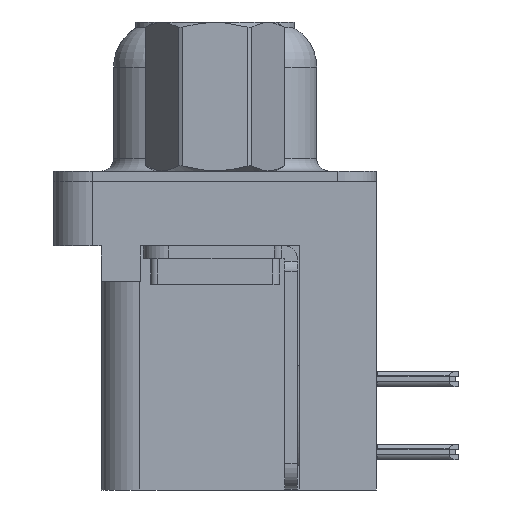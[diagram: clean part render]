
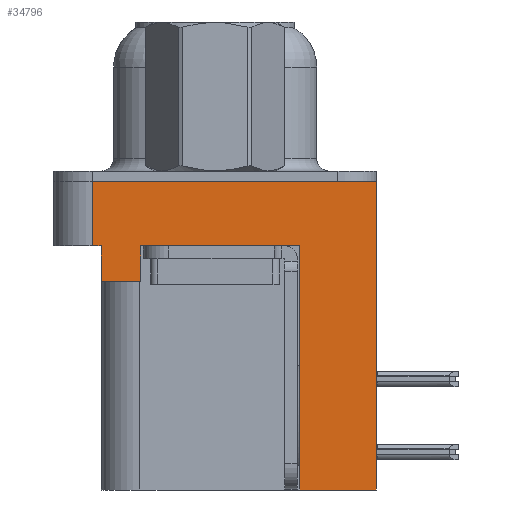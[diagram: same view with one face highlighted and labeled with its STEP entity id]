
A CAD part, left-side view. The second image highlights one B-rep face of the part: STEP entity #34796.
In plain terms, the highlighted planar face has unit normal (-1, 0, 0).
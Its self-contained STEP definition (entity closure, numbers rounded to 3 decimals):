
#203 = VECTOR ( 'NONE', #33293, 1000. ) ;
#661 = VERTEX_POINT ( 'NONE', #14032 ) ;
#701 = LINE ( 'NONE', #36045, #203 ) ;
#833 = LINE ( 'NONE', #17079, #24653 ) ;
#1160 = VERTEX_POINT ( 'NONE', #25653 ) ;
#1817 = VERTEX_POINT ( 'NONE', #3060 ) ;
#1868 = VECTOR ( 'NONE', #26045, 1000. ) ;
#1996 = VECTOR ( 'NONE', #5836, 1000. ) ;
#2116 = ORIENTED_EDGE ( 'NONE', *, *, #36443, .F. ) ;
#2632 = CARTESIAN_POINT ( 'NONE',  ( -3., 4.775, -2.5 ) ) ;
#3060 = CARTESIAN_POINT ( 'NONE',  ( -3., -3.295, -12. ) ) ;
#4125 = DIRECTION ( 'NONE',  ( 0., -1., 0. ) ) ;
#5106 = LINE ( 'NONE', #2632, #1996 ) ;
#5511 = DIRECTION ( 'NONE',  ( 0., 0., 1. ) ) ;
#5622 = ORIENTED_EDGE ( 'NONE', *, *, #32778, .F. ) ;
#5836 = DIRECTION ( 'NONE',  ( 0., 0., 1. ) ) ;
#6064 = FACE_OUTER_BOUND ( 'NONE', #20795, .T. ) ;
#6183 = DIRECTION ( 'NONE',  ( 0., 1., 0. ) ) ;
#6506 = VECTOR ( 'NONE', #8649, 1000. ) ;
#7012 = ORIENTED_EDGE ( 'NONE', *, *, #32223, .T. ) ;
#7039 = VERTEX_POINT ( 'NONE', #19351 ) ;
#7187 = VECTOR ( 'NONE', #5511, 1000. ) ;
#7406 = CARTESIAN_POINT ( 'NONE',  ( -3., -6.275, -2.5 ) ) ;
#8396 = LINE ( 'NONE', #28983, #18297 ) ;
#8625 = VERTEX_POINT ( 'NONE', #19706 ) ;
#8649 = DIRECTION ( 'NONE',  ( 0., 0., 1. ) ) ;
#9551 = VECTOR ( 'NONE', #12035, 1000. ) ;
#9947 = LINE ( 'NONE', #23900, #34202 ) ;
#11908 = CARTESIAN_POINT ( 'NONE',  ( -3., 2.895, -3.9 ) ) ;
#12035 = DIRECTION ( 'NONE',  ( 0., 1., 0. ) ) ;
#12467 = ORIENTED_EDGE ( 'NONE', *, *, #16066, .F. ) ;
#13062 = ORIENTED_EDGE ( 'NONE', *, *, #21105, .F. ) ;
#13386 = CARTESIAN_POINT ( 'NONE',  ( -3., -6.275, -12. ) ) ;
#14032 = CARTESIAN_POINT ( 'NONE',  ( -3., 4.425, -3.9 ) ) ;
#14175 = VECTOR ( 'NONE', #4125, 1000. ) ;
#14277 = ORIENTED_EDGE ( 'NONE', *, *, #25251, .F. ) ;
#14768 = CARTESIAN_POINT ( 'NONE',  ( -3., 4.425, -3.9 ) ) ;
#15149 = CARTESIAN_POINT ( 'NONE',  ( -3., -6.275, 0. ) ) ;
#15582 = ORIENTED_EDGE ( 'NONE', *, *, #23860, .T. ) ;
#16066 = EDGE_CURVE ( 'NONE', #28589, #8625, #5106, .T. ) ;
#16696 = ORIENTED_EDGE ( 'NONE', *, *, #24998, .T. ) ;
#17079 = CARTESIAN_POINT ( 'NONE',  ( -3., -3.295, -12. ) ) ;
#18297 = VECTOR ( 'NONE', #6183, 1000. ) ;
#19138 = LINE ( 'NONE', #15149, #14175 ) ;
#19351 = CARTESIAN_POINT ( 'NONE',  ( -3., 2.895, -3.9 ) ) ;
#19706 = CARTESIAN_POINT ( 'NONE',  ( -3., 4.775, 0. ) ) ;
#19817 = CARTESIAN_POINT ( 'NONE',  ( -3., -6.275, -2.5 ) ) ;
#20795 = EDGE_LOOP ( 'NONE', ( #13062, #12467, #32014, #25478, #14277, #16696, #15582, #5622, #2116, #7012 ) ) ;
#21105 = EDGE_CURVE ( 'NONE', #8625, #31920, #19138, .T. ) ;
#21643 = AXIS2_PLACEMENT_3D ( 'NONE', #7406, #30095, #27323 ) ;
#22109 = VERTEX_POINT ( 'NONE', #13386 ) ;
#22446 = LINE ( 'NONE', #19817, #7187 ) ;
#23860 = EDGE_CURVE ( 'NONE', #30116, #1160, #9947, .T. ) ;
#23900 = CARTESIAN_POINT ( 'NONE',  ( -3., -6.275, -2.5 ) ) ;
#24653 = VECTOR ( 'NONE', #28557, 1000. ) ;
#24717 = PLANE ( 'NONE',  #21643 ) ;
#24763 = LINE ( 'NONE', #11908, #1868 ) ;
#24998 = EDGE_CURVE ( 'NONE', #7039, #30116, #24763, .T. ) ;
#25251 = EDGE_CURVE ( 'NONE', #7039, #661, #36142, .T. ) ;
#25478 = ORIENTED_EDGE ( 'NONE', *, *, #34308, .F. ) ;
#25653 = CARTESIAN_POINT ( 'NONE',  ( -3., -3.295, -2.5 ) ) ;
#26015 = CARTESIAN_POINT ( 'NONE',  ( -3., 4.775, -2.5 ) ) ;
#26045 = DIRECTION ( 'NONE',  ( 0., 0., 1. ) ) ;
#27323 = DIRECTION ( 'NONE',  ( 0., 0., 1. ) ) ;
#27340 = EDGE_CURVE ( 'NONE', #28589, #31208, #701, .T. ) ;
#27624 = LINE ( 'NONE', #29073, #6506 ) ;
#28557 = DIRECTION ( 'NONE',  ( 0., 0., 1. ) ) ;
#28589 = VERTEX_POINT ( 'NONE', #26015 ) ;
#28983 = CARTESIAN_POINT ( 'NONE',  ( -3., -3.295, -12. ) ) ;
#29073 = CARTESIAN_POINT ( 'NONE',  ( -3., 4.425, -3.9 ) ) ;
#29399 = CARTESIAN_POINT ( 'NONE',  ( -3., 4.425, -2.5 ) ) ;
#30095 = DIRECTION ( 'NONE',  ( -1., 0., 0. ) ) ;
#30116 = VERTEX_POINT ( 'NONE', #33924 ) ;
#31208 = VERTEX_POINT ( 'NONE', #29399 ) ;
#31920 = VERTEX_POINT ( 'NONE', #32510 ) ;
#32014 = ORIENTED_EDGE ( 'NONE', *, *, #27340, .T. ) ;
#32223 = EDGE_CURVE ( 'NONE', #22109, #31920, #22446, .T. ) ;
#32510 = CARTESIAN_POINT ( 'NONE',  ( -3., -6.275, 0. ) ) ;
#32778 = EDGE_CURVE ( 'NONE', #1817, #1160, #833, .T. ) ;
#33293 = DIRECTION ( 'NONE',  ( 0., -1., 0. ) ) ;
#33924 = CARTESIAN_POINT ( 'NONE',  ( -3., 2.895, -2.5 ) ) ;
#34202 = VECTOR ( 'NONE', #35394, 1000. ) ;
#34308 = EDGE_CURVE ( 'NONE', #661, #31208, #27624, .T. ) ;
#34796 = ADVANCED_FACE ( 'NONE', ( #6064 ), #24717, .T. ) ;
#35394 = DIRECTION ( 'NONE',  ( 0., -1., 0. ) ) ;
#36045 = CARTESIAN_POINT ( 'NONE',  ( -3., -6.275, -2.5 ) ) ;
#36142 = LINE ( 'NONE', #14768, #9551 ) ;
#36443 = EDGE_CURVE ( 'NONE', #22109, #1817, #8396, .T. ) ;
